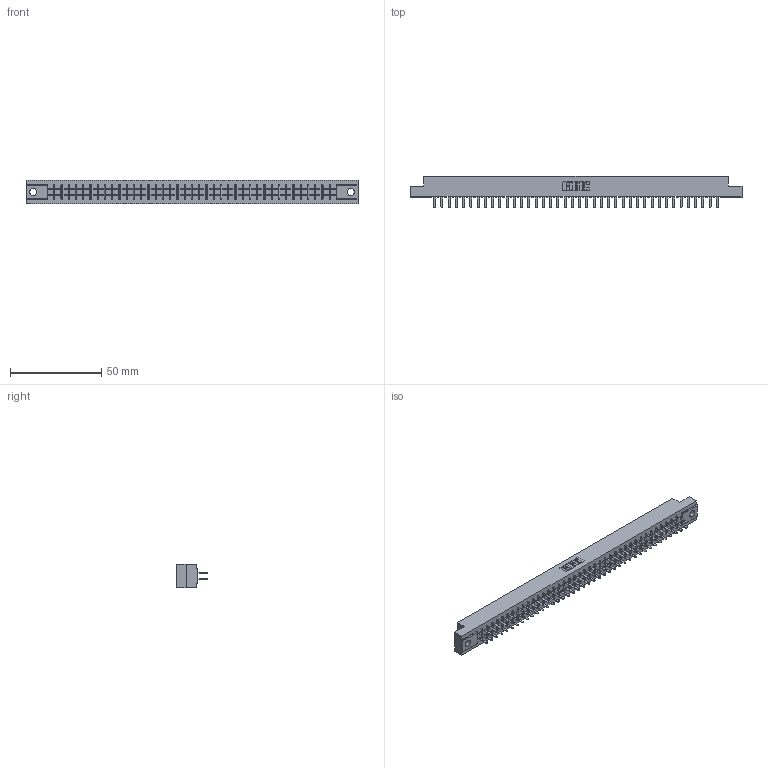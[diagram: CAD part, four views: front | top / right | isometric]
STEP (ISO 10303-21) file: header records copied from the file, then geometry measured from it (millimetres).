
FILE_DESCRIPTION (( 'STEP AP203' ), '1' );
FILE_NAME ('315-080-520-204.STEP', '2019-09-10T23:06:57', ( '' ), ( '' ), 'SwSTEP 2.0', 'SolidWorks 2016', '' );
FILE_SCHEMA (( 'CONFIG_CONTROL_DESIGN' ));
Length unit declared in the file: inch
Products named in the file (3): 315-080-520-204; 305-290-001_520; 305 Part_.156 Dia
Assembly tree (81 placements, depth 2):
  315-080-520-204
    305 Part_.156 Dia
    305-290-001_520  x80
Bounding box: 181.51 x 17.09 x 12.7 mm (x, y, z)
Volume: 18812.7 mm3; surface area: 23784.1 mm2
Topology: 81 solids, 81 shells, 3810 faces, 10872 edges, 7032 vertices
Faces by surface type: plane 2242, cylinder 1408, sphere 160
Entity records: 43851 total; most frequent: CARTESIAN_POINT 7260, ORIENTED_EDGE 7204, DIRECTION 7016, EDGE_CURVE 3602, LINE 2920, VECTOR 2920, VERTEX_POINT 2292, AXIS2_PLACEMENT_3D 2048
